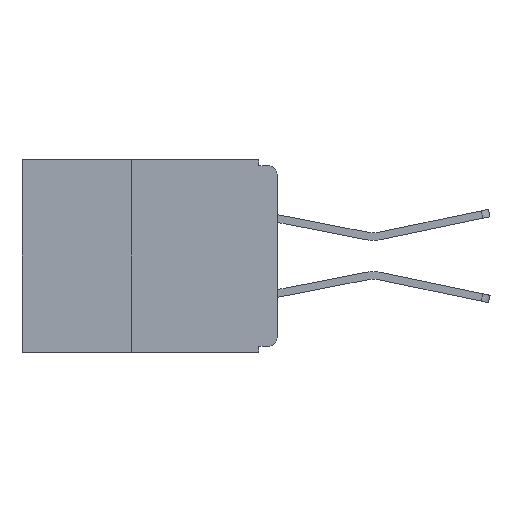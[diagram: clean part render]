
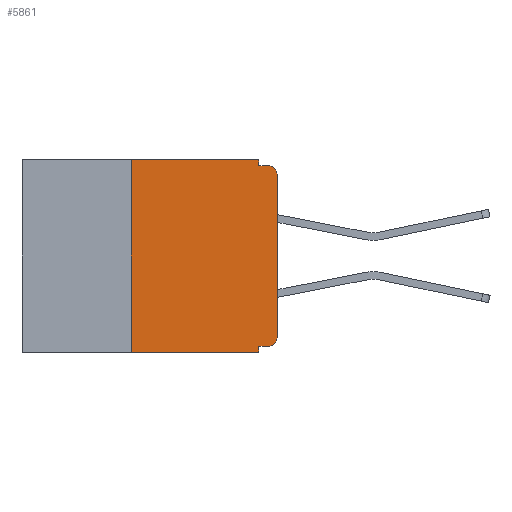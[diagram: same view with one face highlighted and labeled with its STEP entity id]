
A CAD part, left-side view. The second image highlights one B-rep face of the part: STEP entity #5861.
In plain terms, the highlighted planar face has unit normal (-1, 0, 0).
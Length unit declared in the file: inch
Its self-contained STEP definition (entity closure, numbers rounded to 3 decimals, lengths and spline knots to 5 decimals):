
#251 = CARTESIAN_POINT ( 'NONE',  ( 0., 0.031, 0. ) ) ;
#322 = LINE ( 'NONE', #11819, #11304 ) ;
#384 = CARTESIAN_POINT ( 'NONE',  ( 0., 0.25, -0.33 ) ) ;
#392 = FACE_OUTER_BOUND ( 'NONE', #9853, .T. ) ;
#1078 = CARTESIAN_POINT ( 'NONE',  ( 0., 0., -0.025 ) ) ;
#1238 = VERTEX_POINT ( 'NONE', #1895 ) ;
#1442 = EDGE_CURVE ( 'NONE', #5458, #12919, #11646, .T. ) ;
#1457 = CARTESIAN_POINT ( 'NONE',  ( 0., 0., -0.32 ) ) ;
#1496 = DIRECTION ( 'NONE',  ( 0., -1., 0. ) ) ;
#1723 = CARTESIAN_POINT ( 'NONE',  ( 0., 0.25, 0. ) ) ;
#1724 = EDGE_CURVE ( 'NONE', #12919, #4018, #5636, .T. ) ;
#1817 = CARTESIAN_POINT ( 'NONE',  ( 0., 0.015, -0.025 ) ) ;
#1874 = DIRECTION ( 'NONE',  ( 0., 1., 0. ) ) ;
#1876 = DIRECTION ( 'NONE',  ( 0., 0., 1. ) ) ;
#1895 = CARTESIAN_POINT ( 'NONE',  ( 0., 0.031, -0.01 ) ) ;
#2162 = LINE ( 'NONE', #1457, #7201 ) ;
#2506 = EDGE_CURVE ( 'NONE', #9410, #1238, #10335, .T. ) ;
#2558 = VERTEX_POINT ( 'NONE', #11668 ) ;
#2656 = CIRCLE ( 'NONE', #12354, 0.015 ) ;
#2681 = VERTEX_POINT ( 'NONE', #384 ) ;
#2872 = DIRECTION ( 'NONE',  ( 0., 0., -1. ) ) ;
#3016 = LINE ( 'NONE', #11501, #10750 ) ;
#3088 = AXIS2_PLACEMENT_3D ( 'NONE', #1817, #12690, #2872 ) ;
#3134 = ORIENTED_EDGE ( 'NONE', *, *, #11880, .T. ) ;
#3772 = CARTESIAN_POINT ( 'NONE',  ( 0., 0.015, -0.305 ) ) ;
#3773 = ORIENTED_EDGE ( 'NONE', *, *, #5365, .F. ) ;
#3788 = CARTESIAN_POINT ( 'NONE',  ( 0., 0.031, 0. ) ) ;
#4018 = VERTEX_POINT ( 'NONE', #6583 ) ;
#4129 = CARTESIAN_POINT ( 'NONE',  ( 0., 0.25, -0.33 ) ) ;
#4823 = DIRECTION ( 'NONE',  ( 0., 0., -1. ) ) ;
#5020 = ORIENTED_EDGE ( 'NONE', *, *, #1442, .T. ) ;
#5365 = EDGE_CURVE ( 'NONE', #2558, #5724, #2162, .T. ) ;
#5395 = DIRECTION ( 'NONE',  ( 0., 0., 1. ) ) ;
#5458 = VERTEX_POINT ( 'NONE', #13680 ) ;
#5567 = CARTESIAN_POINT ( 'NONE',  ( 0., 0.031, -0.33 ) ) ;
#5636 = CIRCLE ( 'NONE', #3088, 0.015 ) ;
#5649 = EDGE_CURVE ( 'NONE', #2681, #12996, #6705, .T. ) ;
#5724 = VERTEX_POINT ( 'NONE', #11853 ) ;
#5861 = ADVANCED_FACE ( 'NONE', ( #392 ), #10887, .F. ) ;
#5991 = AXIS2_PLACEMENT_3D ( 'NONE', #10904, #10830, #10826 ) ;
#6127 = LINE ( 'NONE', #8169, #9264 ) ;
#6129 = VECTOR ( 'NONE', #5395, 39.37008 ) ;
#6163 = CARTESIAN_POINT ( 'NONE',  ( 0., 0., 0. ) ) ;
#6442 = VECTOR ( 'NONE', #1876, 39.37008 ) ;
#6583 = CARTESIAN_POINT ( 'NONE',  ( 0., 0.015, -0.01 ) ) ;
#6584 = ORIENTED_EDGE ( 'NONE', *, *, #1724, .T. ) ;
#6665 = ORIENTED_EDGE ( 'NONE', *, *, #10941, .F. ) ;
#6705 = LINE ( 'NONE', #12360, #9154 ) ;
#7201 = VECTOR ( 'NONE', #1874, 39.37008 ) ;
#7427 = DIRECTION ( 'NONE',  ( 0., -1., 0. ) ) ;
#8169 = CARTESIAN_POINT ( 'NONE',  ( 0., 0.437, 0. ) ) ;
#8483 = EDGE_CURVE ( 'NONE', #2681, #12633, #9551, .T. ) ;
#8747 = EDGE_CURVE ( 'NONE', #5724, #12996, #322, .T. ) ;
#9154 = VECTOR ( 'NONE', #12544, 39.37008 ) ;
#9264 = VECTOR ( 'NONE', #1496, 39.37008 ) ;
#9293 = DIRECTION ( 'NONE',  ( 0., 0., -1. ) ) ;
#9410 = VERTEX_POINT ( 'NONE', #251 ) ;
#9469 = ORIENTED_EDGE ( 'NONE', *, *, #2506, .F. ) ;
#9551 = LINE ( 'NONE', #4129, #6442 ) ;
#9853 = EDGE_LOOP ( 'NONE', ( #5020, #6584, #6665, #9469, #10797, #11726, #13506, #10045, #3773, #3134 ) ) ;
#10045 = ORIENTED_EDGE ( 'NONE', *, *, #8747, .F. ) ;
#10335 = LINE ( 'NONE', #3788, #13356 ) ;
#10750 = VECTOR ( 'NONE', #7427, 39.37008 ) ;
#10797 = ORIENTED_EDGE ( 'NONE', *, *, #13054, .F. ) ;
#10826 = DIRECTION ( 'NONE',  ( 0., 0., -1. ) ) ;
#10830 = DIRECTION ( 'NONE',  ( 1., 0., 0. ) ) ;
#10887 = PLANE ( 'NONE',  #5991 ) ;
#10904 = CARTESIAN_POINT ( 'NONE',  ( 0., 0.437, 0. ) ) ;
#10941 = EDGE_CURVE ( 'NONE', #1238, #4018, #3016, .T. ) ;
#11031 = DIRECTION ( 'NONE',  ( -1., 0., 0. ) ) ;
#11304 = VECTOR ( 'NONE', #12849, 39.37008 ) ;
#11501 = CARTESIAN_POINT ( 'NONE',  ( 0., 0., -0.01 ) ) ;
#11646 = LINE ( 'NONE', #6163, #6129 ) ;
#11668 = CARTESIAN_POINT ( 'NONE',  ( 0., 0.015, -0.32 ) ) ;
#11726 = ORIENTED_EDGE ( 'NONE', *, *, #8483, .F. ) ;
#11819 = CARTESIAN_POINT ( 'NONE',  ( 0., 0.031, -0.33 ) ) ;
#11853 = CARTESIAN_POINT ( 'NONE',  ( 0., 0.031, -0.32 ) ) ;
#11880 = EDGE_CURVE ( 'NONE', #2558, #5458, #2656, .T. ) ;
#12354 = AXIS2_PLACEMENT_3D ( 'NONE', #3772, #11031, #4823 ) ;
#12360 = CARTESIAN_POINT ( 'NONE',  ( 0., 0.437, -0.33 ) ) ;
#12544 = DIRECTION ( 'NONE',  ( 0., -1., 0. ) ) ;
#12633 = VERTEX_POINT ( 'NONE', #1723 ) ;
#12690 = DIRECTION ( 'NONE',  ( -1., 0., 0. ) ) ;
#12849 = DIRECTION ( 'NONE',  ( 0., 0., -1. ) ) ;
#12919 = VERTEX_POINT ( 'NONE', #1078 ) ;
#12996 = VERTEX_POINT ( 'NONE', #5567 ) ;
#13054 = EDGE_CURVE ( 'NONE', #12633, #9410, #6127, .T. ) ;
#13356 = VECTOR ( 'NONE', #9293, 39.37008 ) ;
#13506 = ORIENTED_EDGE ( 'NONE', *, *, #5649, .T. ) ;
#13680 = CARTESIAN_POINT ( 'NONE',  ( 0., 0., -0.305 ) ) ;
